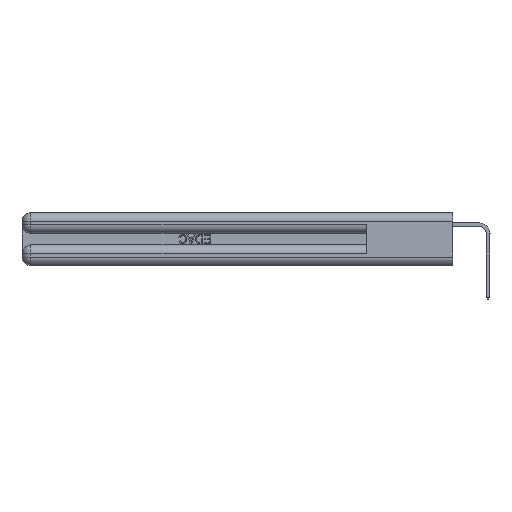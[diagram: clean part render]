
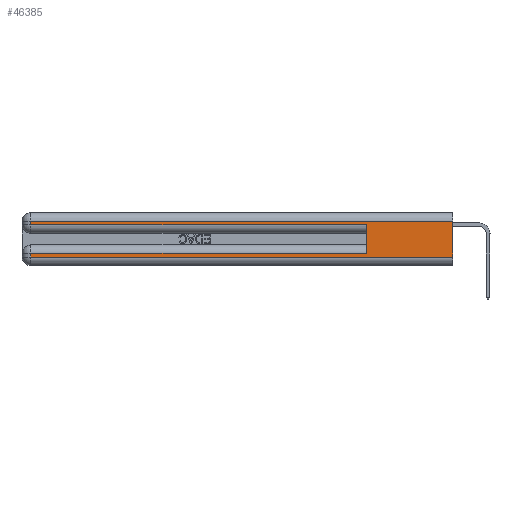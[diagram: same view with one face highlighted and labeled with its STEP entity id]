
A CAD part, left-side view. The second image highlights one B-rep face of the part: STEP entity #46385.
In plain terms, the highlighted planar face has unit normal (-1, 0, 0).
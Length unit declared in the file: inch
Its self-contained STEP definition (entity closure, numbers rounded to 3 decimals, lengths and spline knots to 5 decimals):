
#225 = CARTESIAN_POINT ( 'NONE',  ( 0., 0., 0.31 ) ) ;
#636 = LINE ( 'NONE', #1627, #48183 ) ;
#789 = LINE ( 'NONE', #23017, #18363 ) ;
#955 = DIRECTION ( 'NONE',  ( 0., 0., -1. ) ) ;
#1627 = CARTESIAN_POINT ( 'NONE',  ( 0., 2.94, 0.37 ) ) ;
#3072 = CARTESIAN_POINT ( 'NONE',  ( 0., 0., 0.06 ) ) ;
#3178 = VECTOR ( 'NONE', #955, 39.37008 ) ;
#3239 = EDGE_CURVE ( 'NONE', #42030, #26515, #636, .T. ) ;
#4092 = EDGE_CURVE ( 'NONE', #35786, #25699, #30466, .T. ) ;
#4221 = ORIENTED_EDGE ( 'NONE', *, *, #4092, .T. ) ;
#4351 = DIRECTION ( 'NONE',  ( 0., 1., 0. ) ) ;
#4424 = CARTESIAN_POINT ( 'NONE',  ( 0., 0., 0.31 ) ) ;
#4944 = ORIENTED_EDGE ( 'NONE', *, *, #3239, .T. ) ;
#5057 = EDGE_CURVE ( 'NONE', #41913, #42030, #46825, .T. ) ;
#5280 = ORIENTED_EDGE ( 'NONE', *, *, #5057, .T. ) ;
#5285 = CARTESIAN_POINT ( 'NONE',  ( 0., 0., 0.37 ) ) ;
#9031 = PLANE ( 'NONE',  #39977 ) ;
#9571 = EDGE_LOOP ( 'NONE', ( #13206, #5280, #4944, #43394, #32796, #46564, #4221, #40387 ) ) ;
#10018 = EDGE_CURVE ( 'NONE', #41913, #36319, #24308, .T. ) ;
#10565 = EDGE_CURVE ( 'NONE', #16115, #35786, #789, .T. ) ;
#11552 = CARTESIAN_POINT ( 'NONE',  ( 0., 0., 0.285 ) ) ;
#12808 = DIRECTION ( 'NONE',  ( 0., 0., -1. ) ) ;
#13206 = ORIENTED_EDGE ( 'NONE', *, *, #10018, .F. ) ;
#15332 = DIRECTION ( 'NONE',  ( 0., -1., 0. ) ) ;
#16115 = VERTEX_POINT ( 'NONE', #32116 ) ;
#17712 = VECTOR ( 'NONE', #15332, 39.37008 ) ;
#18363 = VECTOR ( 'NONE', #4351, 39.37008 ) ;
#19634 = CARTESIAN_POINT ( 'NONE',  ( 0., 0., 0.37 ) ) ;
#20435 = VECTOR ( 'NONE', #32759, 39.37008 ) ;
#20511 = LINE ( 'NONE', #3072, #39355 ) ;
#23017 = CARTESIAN_POINT ( 'NONE',  ( 0., 0., 0.085 ) ) ;
#24308 = LINE ( 'NONE', #19634, #3178 ) ;
#25062 = DIRECTION ( 'NONE',  ( 0., -1., 0. ) ) ;
#25213 = CARTESIAN_POINT ( 'NONE',  ( 0., 0.6, 0.145 ) ) ;
#25670 = VECTOR ( 'NONE', #26899, 39.37008 ) ;
#25699 = VERTEX_POINT ( 'NONE', #48620 ) ;
#26003 = FACE_OUTER_BOUND ( 'NONE', #9571, .T. ) ;
#26515 = VERTEX_POINT ( 'NONE', #46261 ) ;
#26899 = DIRECTION ( 'NONE',  ( 0., 1., 0. ) ) ;
#27672 = CARTESIAN_POINT ( 'NONE',  ( 0., 0.6, 0.285 ) ) ;
#28894 = LINE ( 'NONE', #11552, #17712 ) ;
#30401 = EDGE_CURVE ( 'NONE', #26515, #44216, #28894, .T. ) ;
#30466 = LINE ( 'NONE', #40140, #20435 ) ;
#30677 = VECTOR ( 'NONE', #40314, 39.37008 ) ;
#31875 = LINE ( 'NONE', #25213, #30677 ) ;
#32116 = CARTESIAN_POINT ( 'NONE',  ( 0., 0.6, 0.085 ) ) ;
#32759 = DIRECTION ( 'NONE',  ( 0., 0., -1. ) ) ;
#32796 = ORIENTED_EDGE ( 'NONE', *, *, #39696, .F. ) ;
#35786 = VERTEX_POINT ( 'NONE', #46961 ) ;
#36319 = VERTEX_POINT ( 'NONE', #39369 ) ;
#36493 = EDGE_CURVE ( 'NONE', #25699, #36319, #20511, .T. ) ;
#39355 = VECTOR ( 'NONE', #25062, 39.37008 ) ;
#39369 = CARTESIAN_POINT ( 'NONE',  ( 0., 0., 0.06 ) ) ;
#39696 = EDGE_CURVE ( 'NONE', #16115, #44216, #31875, .T. ) ;
#39977 = AXIS2_PLACEMENT_3D ( 'NONE', #5285, #46494, #12808 ) ;
#40140 = CARTESIAN_POINT ( 'NONE',  ( 0., 2.94, 0.37 ) ) ;
#40314 = DIRECTION ( 'NONE',  ( 0., 0., 1. ) ) ;
#40387 = ORIENTED_EDGE ( 'NONE', *, *, #36493, .T. ) ;
#41913 = VERTEX_POINT ( 'NONE', #225 ) ;
#42030 = VERTEX_POINT ( 'NONE', #45985 ) ;
#43394 = ORIENTED_EDGE ( 'NONE', *, *, #30401, .T. ) ;
#44216 = VERTEX_POINT ( 'NONE', #27672 ) ;
#45985 = CARTESIAN_POINT ( 'NONE',  ( 0., 2.94, 0.31 ) ) ;
#46261 = CARTESIAN_POINT ( 'NONE',  ( 0., 2.94, 0.285 ) ) ;
#46385 = ADVANCED_FACE ( 'NONE', ( #26003 ), #9031, .F. ) ;
#46494 = DIRECTION ( 'NONE',  ( 1., 0., 0. ) ) ;
#46564 = ORIENTED_EDGE ( 'NONE', *, *, #10565, .T. ) ;
#46632 = DIRECTION ( 'NONE',  ( 0., 0., -1. ) ) ;
#46825 = LINE ( 'NONE', #4424, #25670 ) ;
#46961 = CARTESIAN_POINT ( 'NONE',  ( 0., 2.94, 0.085 ) ) ;
#48183 = VECTOR ( 'NONE', #46632, 39.37008 ) ;
#48620 = CARTESIAN_POINT ( 'NONE',  ( 0., 2.94, 0.06 ) ) ;
